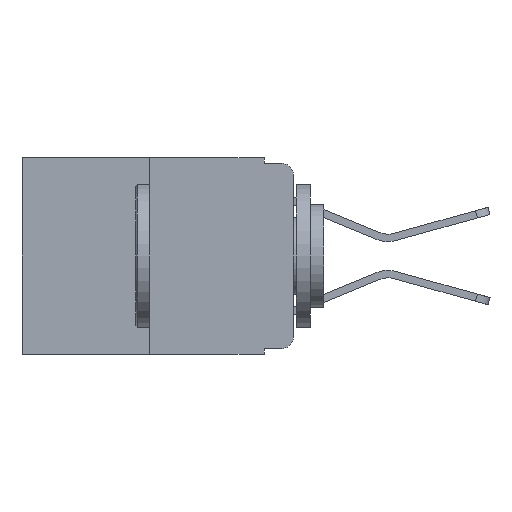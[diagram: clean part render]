
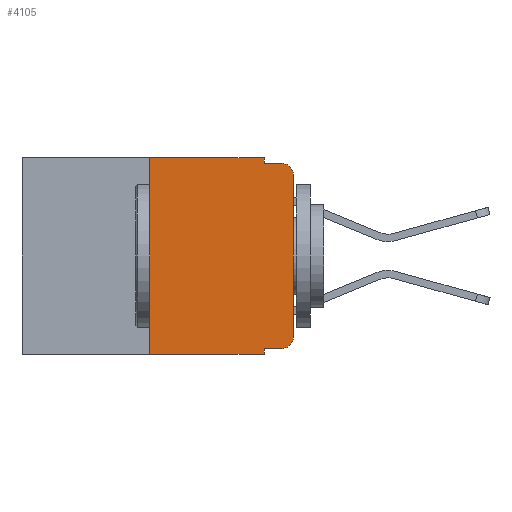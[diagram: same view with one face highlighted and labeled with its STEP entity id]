
A CAD part, left-side view. The second image highlights one B-rep face of the part: STEP entity #4105.
In plain terms, the highlighted planar face has unit normal (-1, 0, 0).
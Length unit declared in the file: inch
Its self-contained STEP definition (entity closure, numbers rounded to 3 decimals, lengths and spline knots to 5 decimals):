
#214 = AXIS2_PLACEMENT_3D ( 'NONE', #11554, #8204, #1499 ) ;
#298 = VECTOR ( 'NONE', #5148, 39.37008 ) ;
#731 = CARTESIAN_POINT ( 'NONE',  ( 0., 0.473, 0. ) ) ;
#1499 = DIRECTION ( 'NONE',  ( 0., 0., -1. ) ) ;
#1841 = ORIENTED_EDGE ( 'NONE', *, *, #8140, .T. ) ;
#2196 = VECTOR ( 'NONE', #15768, 39.37008 ) ;
#2295 = CARTESIAN_POINT ( 'NONE',  ( 0., 0.051, 0. ) ) ;
#2472 = ORIENTED_EDGE ( 'NONE', *, *, #18339, .F. ) ;
#2475 = LINE ( 'NONE', #19741, #12935 ) ;
#2558 = AXIS2_PLACEMENT_3D ( 'NONE', #731, #4636, #16504 ) ;
#3152 = CARTESIAN_POINT ( 'NONE',  ( 0., 0., -0.313 ) ) ;
#4105 = ADVANCED_FACE ( 'NONE', ( #15306 ), #13028, .F. ) ;
#4113 = DIRECTION ( 'NONE',  ( 0., -1., 0. ) ) ;
#4636 = DIRECTION ( 'NONE',  ( 1., 0., 0. ) ) ;
#4672 = LINE ( 'NONE', #13602, #5721 ) ;
#4797 = LINE ( 'NONE', #8523, #298 ) ;
#5058 = VECTOR ( 'NONE', #14192, 39.37008 ) ;
#5148 = DIRECTION ( 'NONE',  ( 0., -1., 0. ) ) ;
#5320 = DIRECTION ( 'NONE',  ( 0., -1., 0. ) ) ;
#5409 = VERTEX_POINT ( 'NONE', #13556 ) ;
#5721 = VECTOR ( 'NONE', #8724, 39.37008 ) ;
#5758 = VERTEX_POINT ( 'NONE', #11665 ) ;
#6010 = CARTESIAN_POINT ( 'NONE',  ( 0., 0.02, -0.313 ) ) ;
#6057 = CARTESIAN_POINT ( 'NONE',  ( 0., 0.473, -0.343 ) ) ;
#6221 = EDGE_CURVE ( 'NONE', #16472, #15579, #2475, .T. ) ;
#6567 = EDGE_CURVE ( 'NONE', #5758, #11316, #19423, .T. ) ;
#6884 = EDGE_CURVE ( 'NONE', #17562, #5409, #4797, .T. ) ;
#7291 = VERTEX_POINT ( 'NONE', #3152 ) ;
#7455 = CARTESIAN_POINT ( 'NONE',  ( 0., 0.051, 0. ) ) ;
#7988 = CARTESIAN_POINT ( 'NONE',  ( 0., 0., -0.03 ) ) ;
#8140 = EDGE_CURVE ( 'NONE', #7291, #13464, #4672, .T. ) ;
#8204 = DIRECTION ( 'NONE',  ( -1., 0., 0. ) ) ;
#8523 = CARTESIAN_POINT ( 'NONE',  ( 0., 0.051, -0.01 ) ) ;
#8724 = DIRECTION ( 'NONE',  ( 0., 0., 1. ) ) ;
#9051 = CARTESIAN_POINT ( 'NONE',  ( 0., 0.02, -0.333 ) ) ;
#9125 = ORIENTED_EDGE ( 'NONE', *, *, #12093, .T. ) ;
#9242 = CARTESIAN_POINT ( 'NONE',  ( 0., 0.051, -0.333 ) ) ;
#9364 = DIRECTION ( 'NONE',  ( -1., 0., 0. ) ) ;
#10254 = CIRCLE ( 'NONE', #214, 0.02 ) ;
#10317 = ORIENTED_EDGE ( 'NONE', *, *, #11140, .F. ) ;
#10713 = VECTOR ( 'NONE', #4113, 39.37008 ) ;
#11038 = DIRECTION ( 'NONE',  ( 0., 0., -1. ) ) ;
#11140 = EDGE_CURVE ( 'NONE', #5758, #16472, #18613, .T. ) ;
#11221 = CARTESIAN_POINT ( 'NONE',  ( 0., 0.051, -0.343 ) ) ;
#11316 = VERTEX_POINT ( 'NONE', #11221 ) ;
#11554 = CARTESIAN_POINT ( 'NONE',  ( 0., 0.02, -0.03 ) ) ;
#11665 = CARTESIAN_POINT ( 'NONE',  ( 0., 0.25, -0.343 ) ) ;
#11969 = CARTESIAN_POINT ( 'NONE',  ( 0., 0.051, 0. ) ) ;
#12093 = EDGE_CURVE ( 'NONE', #13464, #5409, #10254, .T. ) ;
#12376 = DIRECTION ( 'NONE',  ( 0., 0., -1. ) ) ;
#12757 = CIRCLE ( 'NONE', #18133, 0.02 ) ;
#12796 = VECTOR ( 'NONE', #12376, 39.37008 ) ;
#12935 = VECTOR ( 'NONE', #5320, 39.37008 ) ;
#13028 = PLANE ( 'NONE',  #2558 ) ;
#13464 = VERTEX_POINT ( 'NONE', #7988 ) ;
#13556 = CARTESIAN_POINT ( 'NONE',  ( 0., 0.02, -0.01 ) ) ;
#13568 = LINE ( 'NONE', #9242, #10713 ) ;
#13602 = CARTESIAN_POINT ( 'NONE',  ( 0., 0., 0. ) ) ;
#13878 = VERTEX_POINT ( 'NONE', #9051 ) ;
#14192 = DIRECTION ( 'NONE',  ( 0., 0., -1. ) ) ;
#14220 = EDGE_LOOP ( 'NONE', ( #1841, #9125, #18345, #2472, #16693, #10317, #20898, #17818, #17032, #17415 ) ) ;
#14525 = VERTEX_POINT ( 'NONE', #20669 ) ;
#14984 = VECTOR ( 'NONE', #16008, 39.37008 ) ;
#15306 = FACE_OUTER_BOUND ( 'NONE', #14220, .T. ) ;
#15579 = VERTEX_POINT ( 'NONE', #11969 ) ;
#15706 = CARTESIAN_POINT ( 'NONE',  ( 0., 0.25, 0. ) ) ;
#15768 = DIRECTION ( 'NONE',  ( 0., 0., 1. ) ) ;
#15981 = EDGE_CURVE ( 'NONE', #14525, #11316, #20975, .T. ) ;
#16008 = DIRECTION ( 'NONE',  ( 0., -1., 0. ) ) ;
#16472 = VERTEX_POINT ( 'NONE', #19037 ) ;
#16504 = DIRECTION ( 'NONE',  ( 0., 0., -1. ) ) ;
#16693 = ORIENTED_EDGE ( 'NONE', *, *, #6221, .F. ) ;
#17032 = ORIENTED_EDGE ( 'NONE', *, *, #18368, .T. ) ;
#17415 = ORIENTED_EDGE ( 'NONE', *, *, #19013, .T. ) ;
#17448 = LINE ( 'NONE', #2295, #12796 ) ;
#17562 = VERTEX_POINT ( 'NONE', #18268 ) ;
#17818 = ORIENTED_EDGE ( 'NONE', *, *, #15981, .F. ) ;
#18133 = AXIS2_PLACEMENT_3D ( 'NONE', #6010, #9364, #11038 ) ;
#18268 = CARTESIAN_POINT ( 'NONE',  ( 0., 0.051, -0.01 ) ) ;
#18339 = EDGE_CURVE ( 'NONE', #15579, #17562, #17448, .T. ) ;
#18345 = ORIENTED_EDGE ( 'NONE', *, *, #6884, .F. ) ;
#18368 = EDGE_CURVE ( 'NONE', #14525, #13878, #13568, .T. ) ;
#18613 = LINE ( 'NONE', #15706, #2196 ) ;
#19013 = EDGE_CURVE ( 'NONE', #13878, #7291, #12757, .T. ) ;
#19037 = CARTESIAN_POINT ( 'NONE',  ( 0., 0.25, 0. ) ) ;
#19423 = LINE ( 'NONE', #6057, #14984 ) ;
#19741 = CARTESIAN_POINT ( 'NONE',  ( 0., 0.473, 0. ) ) ;
#20669 = CARTESIAN_POINT ( 'NONE',  ( 0., 0.051, -0.333 ) ) ;
#20898 = ORIENTED_EDGE ( 'NONE', *, *, #6567, .T. ) ;
#20975 = LINE ( 'NONE', #7455, #5058 ) ;
